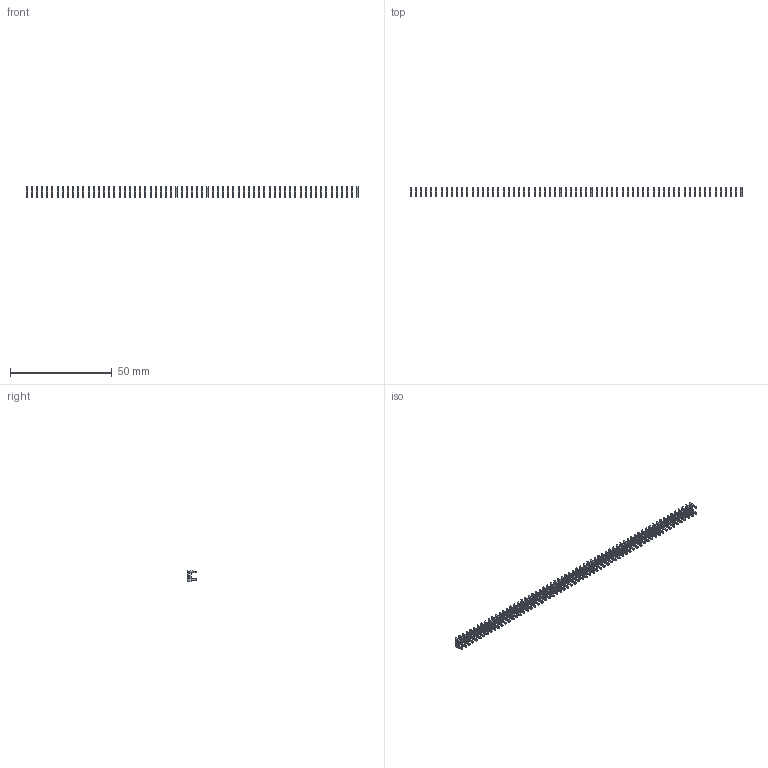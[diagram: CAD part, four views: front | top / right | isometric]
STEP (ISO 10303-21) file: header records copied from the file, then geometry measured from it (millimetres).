
FILE_DESCRIPTION (( 'STEP AP203' ), '1' );
FILE_NAME ('105-065-208-100.STEP', '2020-04-08T01:00:04', ( '' ), ( '' ), 'SwSTEP 2.0', 'SolidWorks 2016', '' );
FILE_SCHEMA (( 'CONFIG_CONTROL_DESIGN' ));
Length unit declared in the file: inch
Products named in the file (2): 100-290-001_100-290-208; 105-065-208-100
Assembly tree (65 placements, depth 2):
  105-065-208-100
    100-290-001_100-290-208  x65
Bounding box: 163.07 x 4.83 x 5.17 mm (x, y, z)
Volume: 447.2 mm3; surface area: 2762.2 mm2
Topology: 65 solids, 65 shells, 1625 faces, 4485 edges, 2990 vertices
Faces by surface type: plane 1430, cylinder 195
Entity records: 3037 total; most frequent: DIRECTION 261, CARTESIAN_POINT 208, COORDINATED_UNIVERSAL_TIME_OFFSET 140, DATE_AND_TIME 140, LOCAL_TIME 140, CALENDAR_DATE 140, ORIENTED_EDGE 138, AXIS2_PLACEMENT_3D 99
